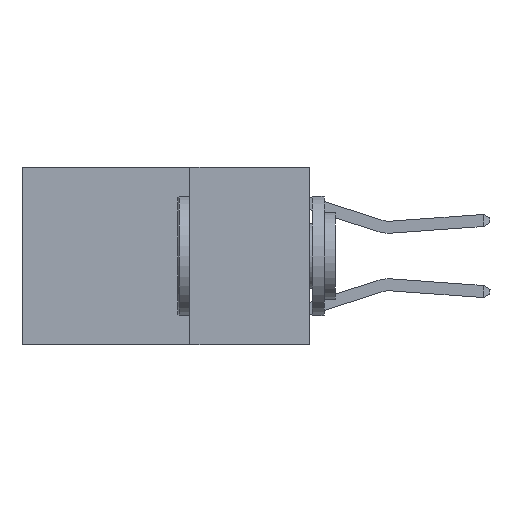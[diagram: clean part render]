
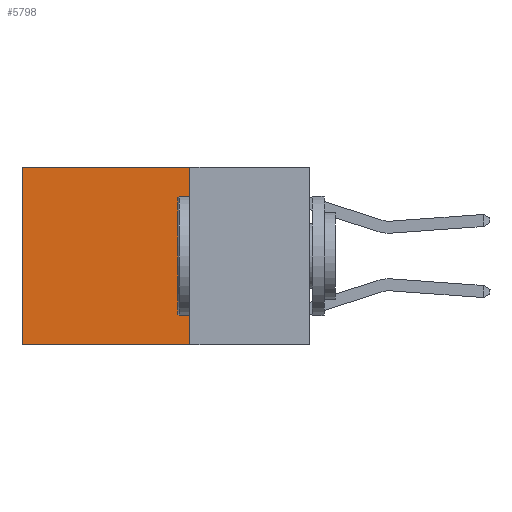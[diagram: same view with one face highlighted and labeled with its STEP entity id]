
A CAD part, left-side view. The second image highlights one B-rep face of the part: STEP entity #5798.
In plain terms, the highlighted planar face has unit normal (-1, 0, 0).
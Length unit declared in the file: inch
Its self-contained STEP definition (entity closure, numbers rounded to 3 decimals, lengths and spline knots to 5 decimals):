
#9 = EDGE_CURVE ( 'NONE', #9870, #18714, #13113, .T. ) ;
#1395 = CARTESIAN_POINT ( 'NONE',  ( 0.2625, 0.25, -0.37 ) ) ;
#2163 = DIRECTION ( 'NONE',  ( 0., 1., 0. ) ) ;
#5182 = CARTESIAN_POINT ( 'NONE',  ( 0.2625, 0.25, 0. ) ) ;
#5772 = CARTESIAN_POINT ( 'NONE',  ( 0.2625, 0.6, -0.37 ) ) ;
#5798 = ADVANCED_FACE ( 'NONE', ( #21193 ), #18318, .F. ) ;
#6267 = VERTEX_POINT ( 'NONE', #5182 ) ;
#6884 = EDGE_LOOP ( 'NONE', ( #15273, #23302, #13301, #7980 ) ) ;
#7980 = ORIENTED_EDGE ( 'NONE', *, *, #18341, .T. ) ;
#8318 = VECTOR ( 'NONE', #2163, 39.37008 ) ;
#8397 = CARTESIAN_POINT ( 'NONE',  ( 0.2625, 0.25, 0. ) ) ;
#9231 = CARTESIAN_POINT ( 'NONE',  ( 0.2625, 0.25, 0. ) ) ;
#9870 = VERTEX_POINT ( 'NONE', #14971 ) ;
#10184 = CARTESIAN_POINT ( 'NONE',  ( 0.2625, 0.6, 0. ) ) ;
#10195 = DIRECTION ( 'NONE',  ( 0., 1., 0. ) ) ;
#10554 = LINE ( 'NONE', #8397, #19639 ) ;
#11027 = DIRECTION ( 'NONE',  ( 0., 0., -1. ) ) ;
#11133 = VERTEX_POINT ( 'NONE', #22651 ) ;
#13113 = LINE ( 'NONE', #1395, #8318 ) ;
#13301 = ORIENTED_EDGE ( 'NONE', *, *, #21963, .F. ) ;
#13339 = DIRECTION ( 'NONE',  ( 0., 0., -1. ) ) ;
#13492 = VECTOR ( 'NONE', #13339, 39.37008 ) ;
#13646 = AXIS2_PLACEMENT_3D ( 'NONE', #9231, #21926, #11027 ) ;
#14971 = CARTESIAN_POINT ( 'NONE',  ( 0.2625, 0.25, -0.37 ) ) ;
#15187 = CARTESIAN_POINT ( 'NONE',  ( 0.2625, 0.25, 0. ) ) ;
#15273 = ORIENTED_EDGE ( 'NONE', *, *, #16500, .T. ) ;
#16500 = EDGE_CURVE ( 'NONE', #11133, #18714, #22749, .T. ) ;
#18318 = PLANE ( 'NONE',  #13646 ) ;
#18341 = EDGE_CURVE ( 'NONE', #6267, #11133, #10554, .T. ) ;
#18714 = VERTEX_POINT ( 'NONE', #5772 ) ;
#19639 = VECTOR ( 'NONE', #10195, 39.37008 ) ;
#21193 = FACE_OUTER_BOUND ( 'NONE', #6884, .T. ) ;
#21926 = DIRECTION ( 'NONE',  ( 1., 0., 0. ) ) ;
#21963 = EDGE_CURVE ( 'NONE', #6267, #9870, #23171, .T. ) ;
#22651 = CARTESIAN_POINT ( 'NONE',  ( 0.2625, 0.6, 0. ) ) ;
#22749 = LINE ( 'NONE', #10184, #23340 ) ;
#22898 = DIRECTION ( 'NONE',  ( 0., 0., -1. ) ) ;
#23171 = LINE ( 'NONE', #15187, #13492 ) ;
#23302 = ORIENTED_EDGE ( 'NONE', *, *, #9, .F. ) ;
#23340 = VECTOR ( 'NONE', #22898, 39.37008 ) ;
